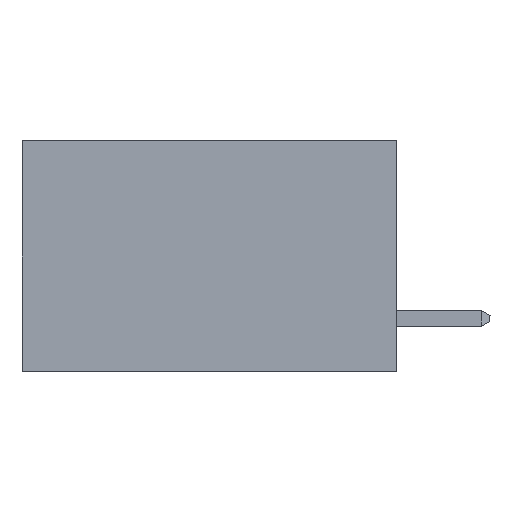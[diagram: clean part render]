
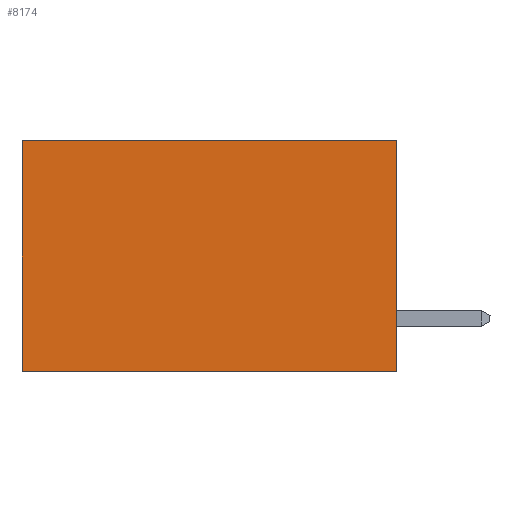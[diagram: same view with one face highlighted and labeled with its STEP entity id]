
A CAD part, left-side view. The second image highlights one B-rep face of the part: STEP entity #8174.
In plain terms, the highlighted planar face has unit normal (-1, 0, 0).
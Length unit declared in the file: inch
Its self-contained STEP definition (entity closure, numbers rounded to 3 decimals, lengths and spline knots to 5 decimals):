
#312 = VERTEX_POINT ( 'NONE', #9514 ) ;
#1307 = ORIENTED_EDGE ( 'NONE', *, *, #12062, .F. ) ;
#1329 = EDGE_LOOP ( 'NONE', ( #21104, #1307, #14742, #13880 ) ) ;
#2214 = DIRECTION ( 'NONE',  ( 0., 0., -1. ) ) ;
#3308 = VECTOR ( 'NONE', #5526, 39.37008 ) ;
#3570 = DIRECTION ( 'NONE',  ( 0., 0., -1. ) ) ;
#3595 = DIRECTION ( 'NONE',  ( 1., 0., 0. ) ) ;
#3655 = CARTESIAN_POINT ( 'NONE',  ( 0.2615, 0., -0.37 ) ) ;
#3751 = PLANE ( 'NONE',  #7053 ) ;
#4397 = LINE ( 'NONE', #7539, #18337 ) ;
#4803 = EDGE_CURVE ( 'NONE', #5826, #23132, #22664, .T. ) ;
#4932 = VECTOR ( 'NONE', #16635, 39.37008 ) ;
#5526 = DIRECTION ( 'NONE',  ( 0., 0., -1. ) ) ;
#5577 = CARTESIAN_POINT ( 'NONE',  ( 0.2615, 0.6, 0. ) ) ;
#5826 = VERTEX_POINT ( 'NONE', #11010 ) ;
#5902 = EDGE_CURVE ( 'NONE', #5826, #9460, #4397, .T. ) ;
#5973 = DIRECTION ( 'NONE',  ( 0., 1., 0. ) ) ;
#6631 = CARTESIAN_POINT ( 'NONE',  ( 0.2615, 0., -0.37 ) ) ;
#7053 = AXIS2_PLACEMENT_3D ( 'NONE', #3655, #3595, #3570 ) ;
#7539 = CARTESIAN_POINT ( 'NONE',  ( 0.2615, 0., 0. ) ) ;
#7661 = FACE_OUTER_BOUND ( 'NONE', #1329, .T. ) ;
#8174 = ADVANCED_FACE ( 'NONE', ( #7661 ), #3751, .F. ) ;
#9460 = VERTEX_POINT ( 'NONE', #5577 ) ;
#9514 = CARTESIAN_POINT ( 'NONE',  ( 0.2615, 0.6, -0.37 ) ) ;
#9734 = LINE ( 'NONE', #14587, #4932 ) ;
#11010 = CARTESIAN_POINT ( 'NONE',  ( 0.2615, 0., 0. ) ) ;
#12062 = EDGE_CURVE ( 'NONE', #23132, #312, #9734, .T. ) ;
#13880 = ORIENTED_EDGE ( 'NONE', *, *, #5902, .T. ) ;
#14099 = CARTESIAN_POINT ( 'NONE',  ( 0.2615, 0., -0.37 ) ) ;
#14587 = CARTESIAN_POINT ( 'NONE',  ( 0.2615, 0., -0.37 ) ) ;
#14742 = ORIENTED_EDGE ( 'NONE', *, *, #4803, .F. ) ;
#14774 = VECTOR ( 'NONE', #2214, 39.37008 ) ;
#14892 = EDGE_CURVE ( 'NONE', #9460, #312, #19630, .T. ) ;
#15044 = CARTESIAN_POINT ( 'NONE',  ( 0.2615, 0.6, -0.37 ) ) ;
#16635 = DIRECTION ( 'NONE',  ( 0., 1., 0. ) ) ;
#18337 = VECTOR ( 'NONE', #5973, 39.37008 ) ;
#19630 = LINE ( 'NONE', #15044, #14774 ) ;
#21104 = ORIENTED_EDGE ( 'NONE', *, *, #14892, .T. ) ;
#22664 = LINE ( 'NONE', #6631, #3308 ) ;
#23132 = VERTEX_POINT ( 'NONE', #14099 ) ;
